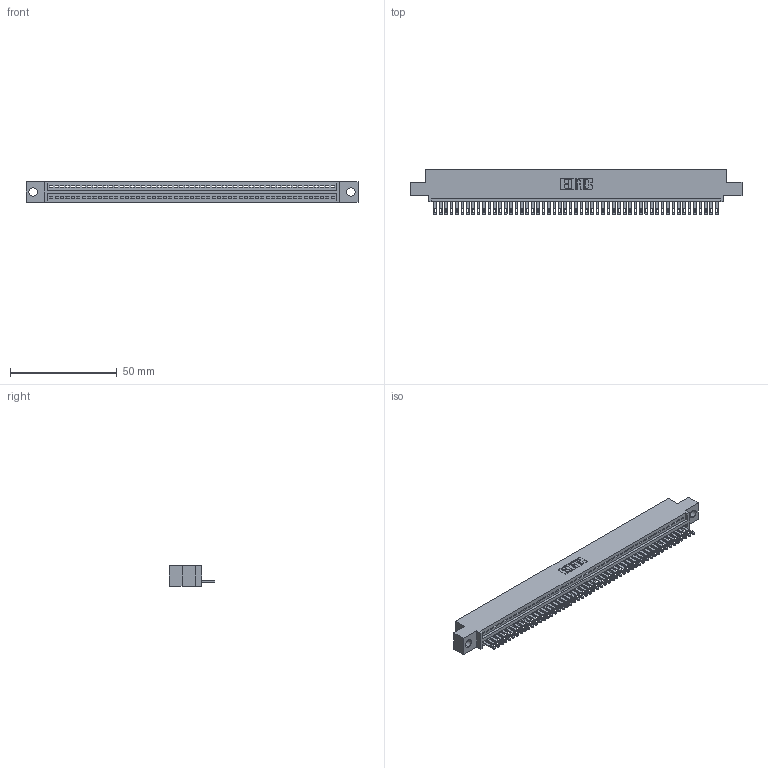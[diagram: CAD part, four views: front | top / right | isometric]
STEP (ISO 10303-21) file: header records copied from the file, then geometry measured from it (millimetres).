
FILE_DESCRIPTION (( 'STEP AP203' ), '1' );
FILE_NAME ('895-053-500-404.STEP', '2020-09-27T12:25:56', ( '' ), ( '' ), 'SwSTEP 2.0', 'SolidWorks 2020', '' );
FILE_SCHEMA (( 'CONFIG_CONTROL_DESIGN' ));
Length unit declared in the file: inch
Products named in the file (3): 845 Part_0.110 Offset - 0.156 Dia-TH; 895-053-500-404; 345-292-001_345-293-100
Assembly tree (54 placements, depth 2):
  895-053-500-404
    845 Part_0.110 Offset - 0.156 Dia-TH
    345-292-001_345-293-100  x53
Bounding box: 155.83 x 21.51 x 9.4 mm (x, y, z)
Volume: 14762.5 mm3; surface area: 19777.2 mm2
Topology: 54 solids, 54 shells, 2992 faces, 9257 edges, 6170 vertices
Faces by surface type: plane 1886, cylinder 1106
Entity records: 38473 total; most frequent: CARTESIAN_POINT 6671, ORIENTED_EDGE 6658, DIRECTION 5811, EDGE_CURVE 3329, VECTOR 2981, LINE 2981, VERTEX_POINT 2218, AXIS2_PLACEMENT_3D 1415
